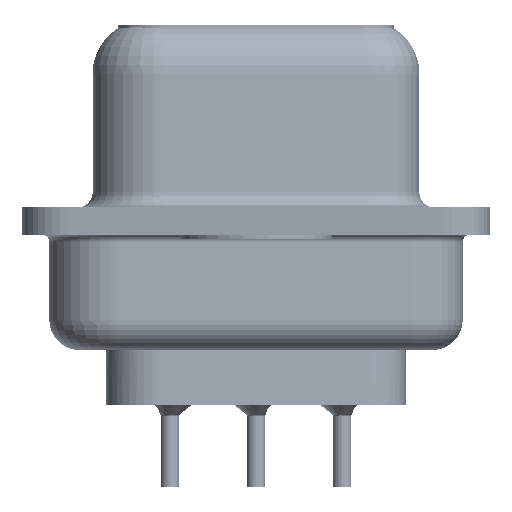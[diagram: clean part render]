
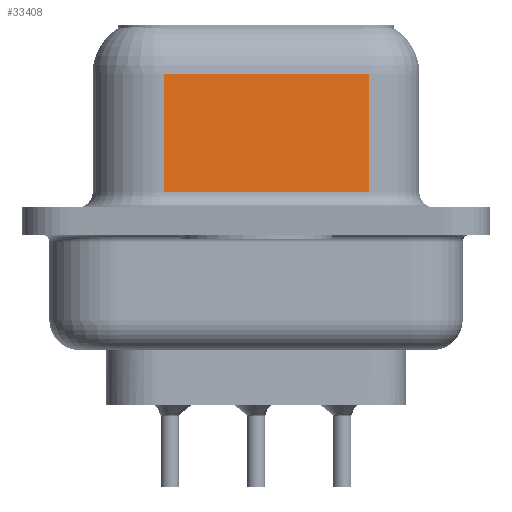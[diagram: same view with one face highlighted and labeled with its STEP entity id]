
A CAD part, left-side view. The second image highlights one B-rep face of the part: STEP entity #33408.
In plain terms, the highlighted planar face has unit normal (-0.985, -0.174, 0).
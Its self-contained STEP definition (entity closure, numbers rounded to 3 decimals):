
#2927 = ORIENTED_EDGE ( 'NONE', *, *, #11675, .T. ) ;
#5693 = PLANE ( 'NONE',  #27206 ) ;
#6725 = ORIENTED_EDGE ( 'NONE', *, *, #38114, .T. ) ;
#6926 = VERTEX_POINT ( 'NONE', #38865 ) ;
#7490 = CARTESIAN_POINT ( 'NONE',  ( 4.43, 3.028, 4.85 ) ) ;
#8945 = DIRECTION ( 'NONE',  ( -0.174, 0.985, 0. ) ) ;
#9181 = CARTESIAN_POINT ( 'NONE',  ( 5.621, -3.722, 0.95 ) ) ;
#10686 = DIRECTION ( 'NONE',  ( 0., 0., -1. ) ) ;
#10805 = CARTESIAN_POINT ( 'NONE',  ( 4.43, 3.028, 0.95 ) ) ;
#10961 = CARTESIAN_POINT ( 'NONE',  ( 5.621, -3.722, 0.95 ) ) ;
#11675 = EDGE_CURVE ( 'NONE', #6926, #32221, #32095, .T. ) ;
#12935 = FACE_OUTER_BOUND ( 'NONE', #19901, .T. ) ;
#13132 = VECTOR ( 'NONE', #10686, 1000. ) ;
#13631 = VERTEX_POINT ( 'NONE', #10805 ) ;
#13912 = DIRECTION ( 'NONE',  ( 0.174, -0.985, 0. ) ) ;
#16950 = VECTOR ( 'NONE', #17465, 1000. ) ;
#17465 = DIRECTION ( 'NONE',  ( 0., 0., -1. ) ) ;
#19367 = LINE ( 'NONE', #10961, #28420 ) ;
#19901 = EDGE_LOOP ( 'NONE', ( #26341, #2927, #6725, #31164 ) ) ;
#22504 = CARTESIAN_POINT ( 'NONE',  ( 5.621, -3.722, 4.85 ) ) ;
#22979 = EDGE_CURVE ( 'NONE', #6926, #38793, #29400, .T. ) ;
#23029 = EDGE_CURVE ( 'NONE', #13631, #38793, #19367, .T. ) ;
#23562 = CARTESIAN_POINT ( 'NONE',  ( 4.43, 3.028, 6.6 ) ) ;
#24006 = VECTOR ( 'NONE', #28359, 1000. ) ;
#26341 = ORIENTED_EDGE ( 'NONE', *, *, #22979, .F. ) ;
#27206 = AXIS2_PLACEMENT_3D ( 'NONE', #36387, #27272, #8945 ) ;
#27272 = DIRECTION ( 'NONE',  ( 0.985, 0.174, 0. ) ) ;
#28359 = DIRECTION ( 'NONE',  ( -0.174, 0.985, 0. ) ) ;
#28420 = VECTOR ( 'NONE', #13912, 1000. ) ;
#29400 = LINE ( 'NONE', #32077, #13132 ) ;
#31164 = ORIENTED_EDGE ( 'NONE', *, *, #23029, .T. ) ;
#32077 = CARTESIAN_POINT ( 'NONE',  ( 5.621, -3.722, 6.6 ) ) ;
#32095 = LINE ( 'NONE', #22504, #24006 ) ;
#32221 = VERTEX_POINT ( 'NONE', #7490 ) ;
#33408 = ADVANCED_FACE ( 'NONE', ( #12935 ), #5693, .F. ) ;
#34142 = LINE ( 'NONE', #23562, #16950 ) ;
#36387 = CARTESIAN_POINT ( 'NONE',  ( 5.621, -3.722, 6.6 ) ) ;
#38114 = EDGE_CURVE ( 'NONE', #32221, #13631, #34142, .T. ) ;
#38793 = VERTEX_POINT ( 'NONE', #9181 ) ;
#38865 = CARTESIAN_POINT ( 'NONE',  ( 5.621, -3.722, 4.85 ) ) ;
